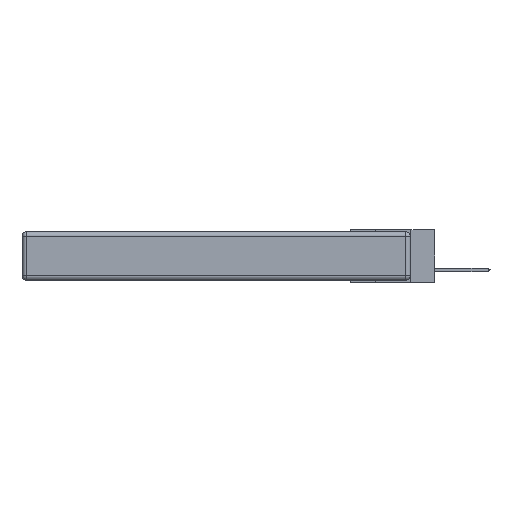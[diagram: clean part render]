
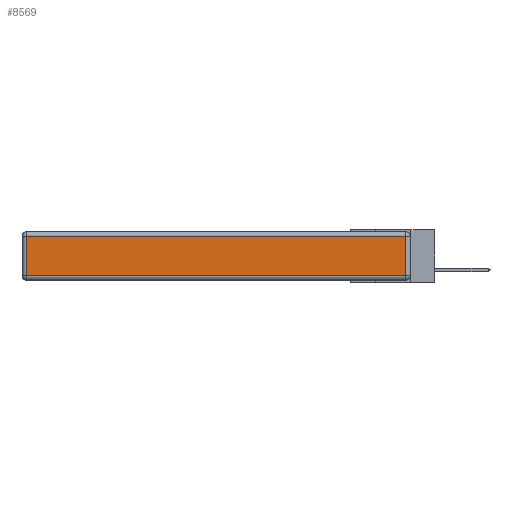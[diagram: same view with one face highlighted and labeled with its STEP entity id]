
A CAD part, left-side view. The second image highlights one B-rep face of the part: STEP entity #8569.
In plain terms, the highlighted planar face has unit normal (-1, 0, 0).
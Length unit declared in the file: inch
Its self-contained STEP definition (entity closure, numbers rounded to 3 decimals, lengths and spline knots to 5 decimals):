
#1470 = VECTOR ( 'NONE', #16805, 39.37008 ) ;
#1560 = LINE ( 'NONE', #2445, #3964 ) ;
#2445 = CARTESIAN_POINT ( 'NONE',  ( 0., 0.03, -0.343 ) ) ;
#2719 = EDGE_CURVE ( 'NONE', #24155, #24182, #25864, .T. ) ;
#3652 = CARTESIAN_POINT ( 'NONE',  ( 0., 0., -0.343 ) ) ;
#3964 = VECTOR ( 'NONE', #4584, 39.37008 ) ;
#4584 = DIRECTION ( 'NONE',  ( 0., 0., 1. ) ) ;
#5765 = CARTESIAN_POINT ( 'NONE',  ( 0., 2.72, -0.343 ) ) ;
#6265 = AXIS2_PLACEMENT_3D ( 'NONE', #3652, #23173, #12335 ) ;
#6541 = EDGE_CURVE ( 'NONE', #24182, #15844, #23450, .T. ) ;
#6607 = VECTOR ( 'NONE', #23833, 39.37008 ) ;
#7728 = EDGE_CURVE ( 'NONE', #15844, #16192, #11609, .T. ) ;
#8148 = ORIENTED_EDGE ( 'NONE', *, *, #10957, .T. ) ;
#8569 = ADVANCED_FACE ( 'NONE', ( #9517 ), #25240, .T. ) ;
#9517 = FACE_OUTER_BOUND ( 'NONE', #24051, .T. ) ;
#9934 = CARTESIAN_POINT ( 'NONE',  ( 0., 2.72, -0.03 ) ) ;
#9965 = CARTESIAN_POINT ( 'NONE',  ( 0., 2.72, -0.313 ) ) ;
#10957 = EDGE_CURVE ( 'NONE', #16192, #24155, #1560, .T. ) ;
#10980 = ORIENTED_EDGE ( 'NONE', *, *, #6541, .T. ) ;
#11609 = LINE ( 'NONE', #27071, #12604 ) ;
#12335 = DIRECTION ( 'NONE',  ( 0., 0., 1. ) ) ;
#12604 = VECTOR ( 'NONE', #13984, 39.37008 ) ;
#13692 = ORIENTED_EDGE ( 'NONE', *, *, #7728, .T. ) ;
#13984 = DIRECTION ( 'NONE',  ( 0., -1., 0. ) ) ;
#14367 = CARTESIAN_POINT ( 'NONE',  ( 0., 0.03, -0.313 ) ) ;
#15844 = VERTEX_POINT ( 'NONE', #9965 ) ;
#16192 = VERTEX_POINT ( 'NONE', #14367 ) ;
#16805 = DIRECTION ( 'NONE',  ( 0., 0., -1. ) ) ;
#22383 = CARTESIAN_POINT ( 'NONE',  ( 0., 0.03, -0.03 ) ) ;
#23173 = DIRECTION ( 'NONE',  ( -1., 0., 0. ) ) ;
#23450 = LINE ( 'NONE', #5765, #1470 ) ;
#23833 = DIRECTION ( 'NONE',  ( 0., 1., 0. ) ) ;
#24051 = EDGE_LOOP ( 'NONE', ( #13692, #8148, #26452, #10980 ) ) ;
#24155 = VERTEX_POINT ( 'NONE', #22383 ) ;
#24182 = VERTEX_POINT ( 'NONE', #9934 ) ;
#25240 = PLANE ( 'NONE',  #6265 ) ;
#25864 = LINE ( 'NONE', #27530, #6607 ) ;
#26452 = ORIENTED_EDGE ( 'NONE', *, *, #2719, .T. ) ;
#27071 = CARTESIAN_POINT ( 'NONE',  ( 0., 0., -0.313 ) ) ;
#27530 = CARTESIAN_POINT ( 'NONE',  ( 0., 2.75, -0.03 ) ) ;
